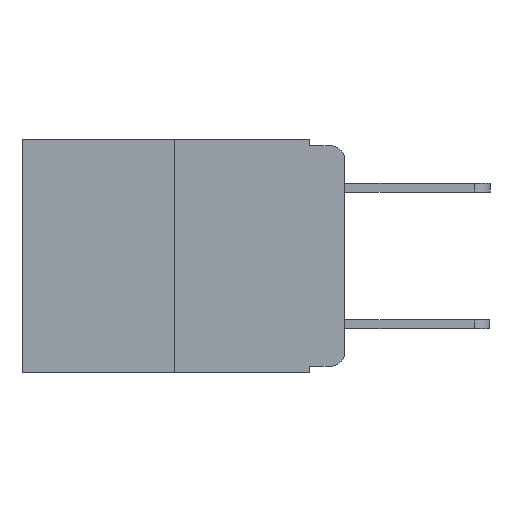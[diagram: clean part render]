
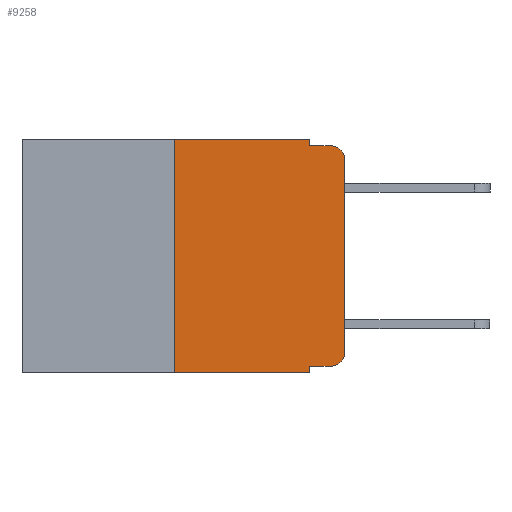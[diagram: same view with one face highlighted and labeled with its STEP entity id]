
A CAD part, left-side view. The second image highlights one B-rep face of the part: STEP entity #9258.
In plain terms, the highlighted planar face has unit normal (-1, 0, 0).
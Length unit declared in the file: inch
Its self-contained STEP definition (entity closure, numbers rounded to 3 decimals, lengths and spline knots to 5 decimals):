
#281 = DIRECTION ( 'NONE',  ( 0., -1., 0. ) ) ;
#321 = EDGE_CURVE ( 'NONE', #3018, #10262, #9538, .T. ) ;
#339 = DIRECTION ( 'NONE',  ( 0., -1., 0. ) ) ;
#845 = VECTOR ( 'NONE', #6234, 39.37008 ) ;
#947 = LINE ( 'NONE', #1687, #7750 ) ;
#1304 = CARTESIAN_POINT ( 'NONE',  ( 0., 0.473, -0.343 ) ) ;
#1372 = VERTEX_POINT ( 'NONE', #3558 ) ;
#1420 = ORIENTED_EDGE ( 'NONE', *, *, #7759, .F. ) ;
#1560 = CARTESIAN_POINT ( 'NONE',  ( 0., 0.051, 0. ) ) ;
#1687 = CARTESIAN_POINT ( 'NONE',  ( 0., 0.051, -0.01 ) ) ;
#1779 = EDGE_CURVE ( 'NONE', #10262, #4357, #947, .T. ) ;
#1795 = VECTOR ( 'NONE', #281, 39.37008 ) ;
#1830 = CARTESIAN_POINT ( 'NONE',  ( 0., 0.02, -0.313 ) ) ;
#2376 = CARTESIAN_POINT ( 'NONE',  ( 0., 0.02, -0.03 ) ) ;
#2478 = CARTESIAN_POINT ( 'NONE',  ( 0., 0.02, -0.01 ) ) ;
#2489 = EDGE_CURVE ( 'NONE', #1372, #4357, #9317, .T. ) ;
#2506 = CARTESIAN_POINT ( 'NONE',  ( 0., 0.051, -0.333 ) ) ;
#2575 = LINE ( 'NONE', #5367, #7569 ) ;
#2856 = DIRECTION ( 'NONE',  ( 0., 0., -1. ) ) ;
#2932 = VECTOR ( 'NONE', #6335, 39.37008 ) ;
#3018 = VERTEX_POINT ( 'NONE', #5001 ) ;
#3101 = VERTEX_POINT ( 'NONE', #7106 ) ;
#3139 = EDGE_CURVE ( 'NONE', #3101, #1372, #2575, .T. ) ;
#3199 = ORIENTED_EDGE ( 'NONE', *, *, #2489, .T. ) ;
#3279 = CARTESIAN_POINT ( 'NONE',  ( 0., 0.051, -0.333 ) ) ;
#3349 = DIRECTION ( 'NONE',  ( 0., 0., -1. ) ) ;
#3504 = CARTESIAN_POINT ( 'NONE',  ( 0., 0.473, 0. ) ) ;
#3558 = CARTESIAN_POINT ( 'NONE',  ( 0., 0., -0.03 ) ) ;
#3756 = CARTESIAN_POINT ( 'NONE',  ( 0., 0.02, -0.333 ) ) ;
#3799 = ORIENTED_EDGE ( 'NONE', *, *, #321, .F. ) ;
#4320 = VERTEX_POINT ( 'NONE', #6285 ) ;
#4355 = CARTESIAN_POINT ( 'NONE',  ( 0., 0.25, 0. ) ) ;
#4357 = VERTEX_POINT ( 'NONE', #2478 ) ;
#4536 = DIRECTION ( 'NONE',  ( 0., 0., -1. ) ) ;
#4565 = CARTESIAN_POINT ( 'NONE',  ( 0., 0.473, 0. ) ) ;
#4604 = DIRECTION ( 'NONE',  ( 1., 0., 0. ) ) ;
#4605 = VERTEX_POINT ( 'NONE', #8411 ) ;
#4632 = EDGE_CURVE ( 'NONE', #6101, #3101, #5062, .T. ) ;
#4796 = ORIENTED_EDGE ( 'NONE', *, *, #3139, .T. ) ;
#5001 = CARTESIAN_POINT ( 'NONE',  ( 0., 0.051, 0. ) ) ;
#5047 = LINE ( 'NONE', #2506, #9998 ) ;
#5062 = CIRCLE ( 'NONE', #5913, 0.02 ) ;
#5181 = VECTOR ( 'NONE', #4536, 39.37008 ) ;
#5244 = EDGE_CURVE ( 'NONE', #7596, #6101, #5047, .T. ) ;
#5283 = AXIS2_PLACEMENT_3D ( 'NONE', #4565, #4604, #11061 ) ;
#5353 = VERTEX_POINT ( 'NONE', #5430 ) ;
#5367 = CARTESIAN_POINT ( 'NONE',  ( 0., 0., 0. ) ) ;
#5411 = AXIS2_PLACEMENT_3D ( 'NONE', #2376, #8922, #3349 ) ;
#5430 = CARTESIAN_POINT ( 'NONE',  ( 0., 0.25, -0.343 ) ) ;
#5897 = EDGE_CURVE ( 'NONE', #7596, #4320, #7680, .T. ) ;
#5913 = AXIS2_PLACEMENT_3D ( 'NONE', #1830, #8447, #2856 ) ;
#5993 = ORIENTED_EDGE ( 'NONE', *, *, #1779, .F. ) ;
#6101 = VERTEX_POINT ( 'NONE', #3756 ) ;
#6234 = DIRECTION ( 'NONE',  ( 0., 0., 1. ) ) ;
#6285 = CARTESIAN_POINT ( 'NONE',  ( 0., 0.051, -0.343 ) ) ;
#6291 = ORIENTED_EDGE ( 'NONE', *, *, #9143, .F. ) ;
#6335 = DIRECTION ( 'NONE',  ( 0., -1., 0. ) ) ;
#6871 = ORIENTED_EDGE ( 'NONE', *, *, #5897, .F. ) ;
#7106 = CARTESIAN_POINT ( 'NONE',  ( 0., 0., -0.313 ) ) ;
#7155 = CARTESIAN_POINT ( 'NONE',  ( 0., 0.051, 0. ) ) ;
#7181 = LINE ( 'NONE', #1304, #1795 ) ;
#7371 = VECTOR ( 'NONE', #9642, 39.37008 ) ;
#7569 = VECTOR ( 'NONE', #8146, 39.37008 ) ;
#7596 = VERTEX_POINT ( 'NONE', #3279 ) ;
#7680 = LINE ( 'NONE', #1560, #5181 ) ;
#7750 = VECTOR ( 'NONE', #8334, 39.37008 ) ;
#7759 = EDGE_CURVE ( 'NONE', #5353, #4605, #7948, .T. ) ;
#7909 = LINE ( 'NONE', #3504, #2932 ) ;
#7948 = LINE ( 'NONE', #4355, #845 ) ;
#8146 = DIRECTION ( 'NONE',  ( 0., 0., 1. ) ) ;
#8334 = DIRECTION ( 'NONE',  ( 0., -1., 0. ) ) ;
#8411 = CARTESIAN_POINT ( 'NONE',  ( 0., 0.25, 0. ) ) ;
#8447 = DIRECTION ( 'NONE',  ( -1., 0., 0. ) ) ;
#8922 = DIRECTION ( 'NONE',  ( -1., 0., 0. ) ) ;
#9023 = ORIENTED_EDGE ( 'NONE', *, *, #10458, .T. ) ;
#9143 = EDGE_CURVE ( 'NONE', #4605, #3018, #7909, .T. ) ;
#9258 = ADVANCED_FACE ( 'NONE', ( #11613 ), #10158, .F. ) ;
#9317 = CIRCLE ( 'NONE', #5411, 0.02 ) ;
#9538 = LINE ( 'NONE', #7155, #7371 ) ;
#9613 = ORIENTED_EDGE ( 'NONE', *, *, #4632, .T. ) ;
#9642 = DIRECTION ( 'NONE',  ( 0., 0., -1. ) ) ;
#9687 = CARTESIAN_POINT ( 'NONE',  ( 0., 0.051, -0.01 ) ) ;
#9998 = VECTOR ( 'NONE', #339, 39.37008 ) ;
#10158 = PLANE ( 'NONE',  #5283 ) ;
#10262 = VERTEX_POINT ( 'NONE', #9687 ) ;
#10458 = EDGE_CURVE ( 'NONE', #5353, #4320, #7181, .T. ) ;
#10963 = EDGE_LOOP ( 'NONE', ( #4796, #3199, #5993, #3799, #6291, #1420, #9023, #6871, #11722, #9613 ) ) ;
#11061 = DIRECTION ( 'NONE',  ( 0., 0., -1. ) ) ;
#11613 = FACE_OUTER_BOUND ( 'NONE', #10963, .T. ) ;
#11722 = ORIENTED_EDGE ( 'NONE', *, *, #5244, .T. ) ;
